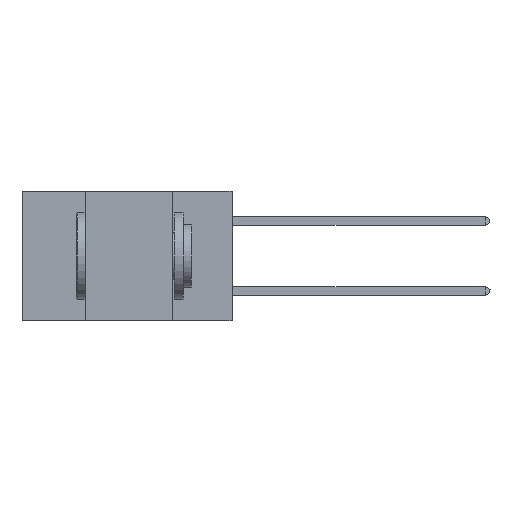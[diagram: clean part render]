
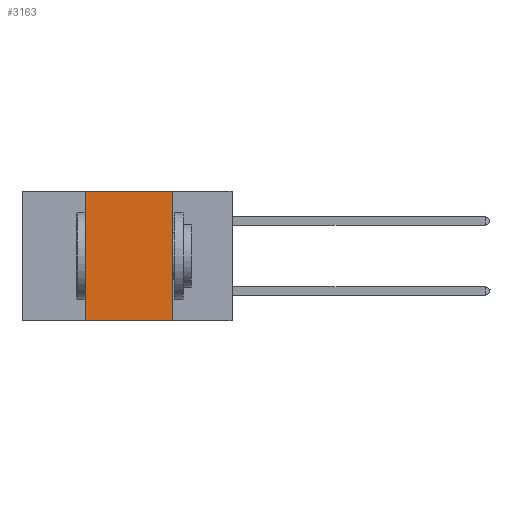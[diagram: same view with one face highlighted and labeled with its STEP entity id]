
A CAD part, left-side view. The second image highlights one B-rep face of the part: STEP entity #3163.
In plain terms, the highlighted planar face has unit normal (-1, 0, 0).
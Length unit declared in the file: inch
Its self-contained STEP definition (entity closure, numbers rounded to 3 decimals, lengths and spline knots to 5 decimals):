
#593 = CARTESIAN_POINT ( 'NONE',  ( 0., 0.17, -0.37 ) ) ;
#835 = VERTEX_POINT ( 'NONE', #1979 ) ;
#1705 = DIRECTION ( 'NONE',  ( 0., 0., 1. ) ) ;
#1845 = ORIENTED_EDGE ( 'NONE', *, *, #12657, .F. ) ;
#1978 = CARTESIAN_POINT ( 'NONE',  ( 0., 0.6, 0. ) ) ;
#1979 = CARTESIAN_POINT ( 'NONE',  ( 0., 0.42, -0.37 ) ) ;
#2723 = VECTOR ( 'NONE', #1705, 39.37008 ) ;
#3075 = VECTOR ( 'NONE', #5360, 39.37008 ) ;
#3141 = ORIENTED_EDGE ( 'NONE', *, *, #4676, .T. ) ;
#3163 = ADVANCED_FACE ( 'NONE', ( #9914 ), #12307, .F. ) ;
#3194 = DIRECTION ( 'NONE',  ( 1., 0., 0. ) ) ;
#4038 = CARTESIAN_POINT ( 'NONE',  ( 0., 0.17, 0. ) ) ;
#4147 = CARTESIAN_POINT ( 'NONE',  ( 0., 0.6, -0.37 ) ) ;
#4676 = EDGE_CURVE ( 'NONE', #835, #5774, #7520, .T. ) ;
#5360 = DIRECTION ( 'NONE',  ( 0., 0., -1. ) ) ;
#5774 = VERTEX_POINT ( 'NONE', #593 ) ;
#5784 = CARTESIAN_POINT ( 'NONE',  ( 0., 0.42, 0. ) ) ;
#6143 = ORIENTED_EDGE ( 'NONE', *, *, #8260, .F. ) ;
#7520 = LINE ( 'NONE', #4147, #12380 ) ;
#7577 = CARTESIAN_POINT ( 'NONE',  ( 0., 0.6, 0. ) ) ;
#8260 = EDGE_CURVE ( 'NONE', #14826, #5774, #12682, .T. ) ;
#8599 = CARTESIAN_POINT ( 'NONE',  ( 0., 0.42, 0. ) ) ;
#9217 = EDGE_LOOP ( 'NONE', ( #6143, #1845, #11409, #3141 ) ) ;
#9731 = EDGE_CURVE ( 'NONE', #835, #9913, #10626, .T. ) ;
#9913 = VERTEX_POINT ( 'NONE', #8599 ) ;
#9914 = FACE_OUTER_BOUND ( 'NONE', #9217, .T. ) ;
#10310 = DIRECTION ( 'NONE',  ( 0., -1., 0. ) ) ;
#10626 = LINE ( 'NONE', #5784, #2723 ) ;
#11396 = CARTESIAN_POINT ( 'NONE',  ( 0., 0.17, 0. ) ) ;
#11409 = ORIENTED_EDGE ( 'NONE', *, *, #9731, .F. ) ;
#11572 = AXIS2_PLACEMENT_3D ( 'NONE', #1978, #3194, #14091 ) ;
#12307 = PLANE ( 'NONE',  #11572 ) ;
#12380 = VECTOR ( 'NONE', #14691, 39.37008 ) ;
#12447 = VECTOR ( 'NONE', #10310, 39.37008 ) ;
#12657 = EDGE_CURVE ( 'NONE', #9913, #14826, #16462, .T. ) ;
#12682 = LINE ( 'NONE', #4038, #3075 ) ;
#14091 = DIRECTION ( 'NONE',  ( 0., 0., -1. ) ) ;
#14691 = DIRECTION ( 'NONE',  ( 0., -1., 0. ) ) ;
#14826 = VERTEX_POINT ( 'NONE', #11396 ) ;
#16462 = LINE ( 'NONE', #7577, #12447 ) ;
